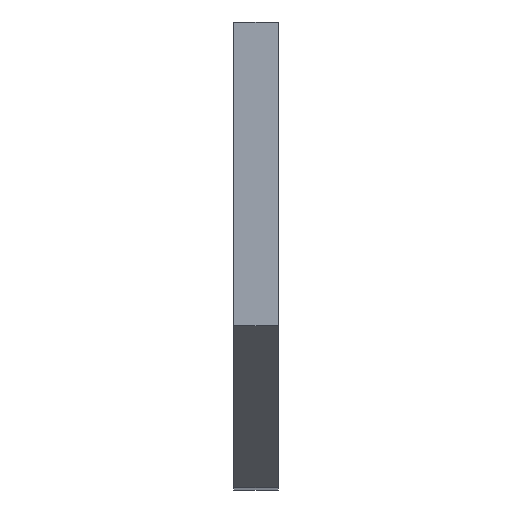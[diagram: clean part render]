
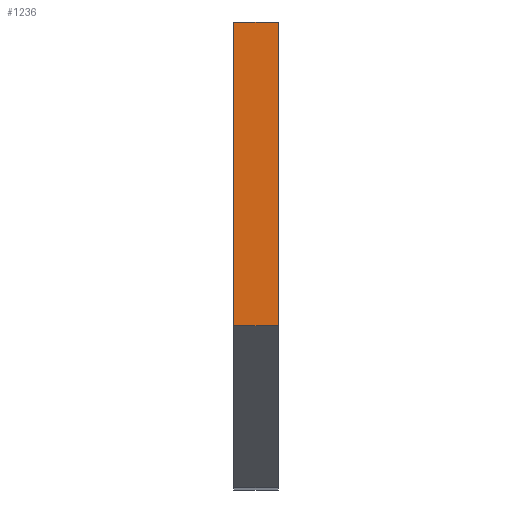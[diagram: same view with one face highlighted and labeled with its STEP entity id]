
A CAD part, top view. The second image highlights one B-rep face of the part: STEP entity #1236.
In plain terms, the highlighted planar face has unit normal (0, 0, 1).
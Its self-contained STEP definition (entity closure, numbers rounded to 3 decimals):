
#54 = PLANE ( 'NONE',  #1128 ) ;
#55 = VERTEX_POINT ( 'NONE', #1084 ) ;
#70 = VERTEX_POINT ( 'NONE', #1077 ) ;
#98 = ORIENTED_EDGE ( 'NONE', *, *, #1006, .T. ) ;
#149 = DIRECTION ( 'NONE',  ( 1., 0., 0. ) ) ;
#156 = CARTESIAN_POINT ( 'NONE',  ( -3.175, 11.608, 0. ) ) ;
#186 = DIRECTION ( 'NONE',  ( 0., 0., 1. ) ) ;
#208 = DIRECTION ( 'NONE',  ( 1., 0., 0. ) ) ;
#210 = CARTESIAN_POINT ( 'NONE',  ( -3.175, 33.426, 0. ) ) ;
#230 = CARTESIAN_POINT ( 'NONE',  ( -3.175, 33.426, 0. ) ) ;
#261 = VECTOR ( 'NONE', #703, 1000. ) ;
#265 = VERTEX_POINT ( 'NONE', #817 ) ;
#294 = EDGE_CURVE ( 'NONE', #55, #70, #303, .T. ) ;
#303 = LINE ( 'NONE', #751, #261 ) ;
#333 = LINE ( 'NONE', #1010, #1110 ) ;
#422 = EDGE_LOOP ( 'NONE', ( #711, #688, #98, #865 ) ) ;
#649 = CARTESIAN_POINT ( 'NONE',  ( -3.175, 0., 0. ) ) ;
#688 = ORIENTED_EDGE ( 'NONE', *, *, #899, .F. ) ;
#703 = DIRECTION ( 'NONE',  ( 0., -1., 0. ) ) ;
#711 = ORIENTED_EDGE ( 'NONE', *, *, #294, .F. ) ;
#717 = DIRECTION ( 'NONE',  ( 0., -1., 0. ) ) ;
#751 = CARTESIAN_POINT ( 'NONE',  ( 0., 0., 0. ) ) ;
#755 = VECTOR ( 'NONE', #149, 1000. ) ;
#817 = CARTESIAN_POINT ( 'NONE',  ( -3.175, 11.608, 0. ) ) ;
#825 = LINE ( 'NONE', #210, #1016 ) ;
#865 = ORIENTED_EDGE ( 'NONE', *, *, #906, .T. ) ;
#899 = EDGE_CURVE ( 'NONE', #1032, #55, #825, .T. ) ;
#906 = EDGE_CURVE ( 'NONE', #265, #70, #998, .T. ) ;
#961 = DIRECTION ( 'NONE',  ( 0., -1., 0. ) ) ;
#998 = LINE ( 'NONE', #156, #755 ) ;
#1006 = EDGE_CURVE ( 'NONE', #1032, #265, #333, .T. ) ;
#1010 = CARTESIAN_POINT ( 'NONE',  ( -3.175, 0., 0. ) ) ;
#1016 = VECTOR ( 'NONE', #208, 1000. ) ;
#1032 = VERTEX_POINT ( 'NONE', #230 ) ;
#1077 = CARTESIAN_POINT ( 'NONE',  ( 0., 11.608, 0. ) ) ;
#1084 = CARTESIAN_POINT ( 'NONE',  ( 0., 33.426, 0. ) ) ;
#1096 = FACE_OUTER_BOUND ( 'NONE', #422, .T. ) ;
#1110 = VECTOR ( 'NONE', #717, 1000. ) ;
#1128 = AXIS2_PLACEMENT_3D ( 'NONE', #649, #186, #961 ) ;
#1236 = ADVANCED_FACE ( 'NONE', ( #1096 ), #54, .T. ) ;
